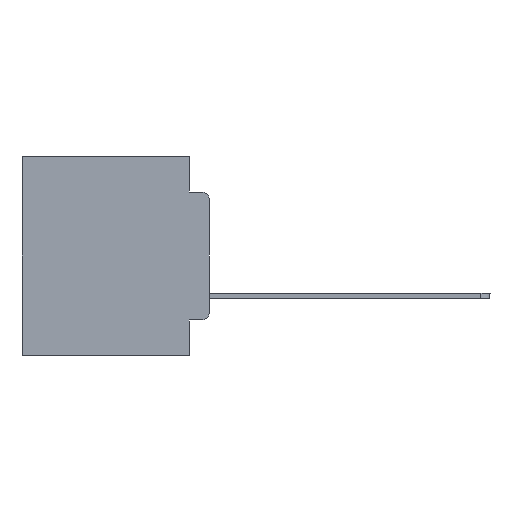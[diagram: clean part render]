
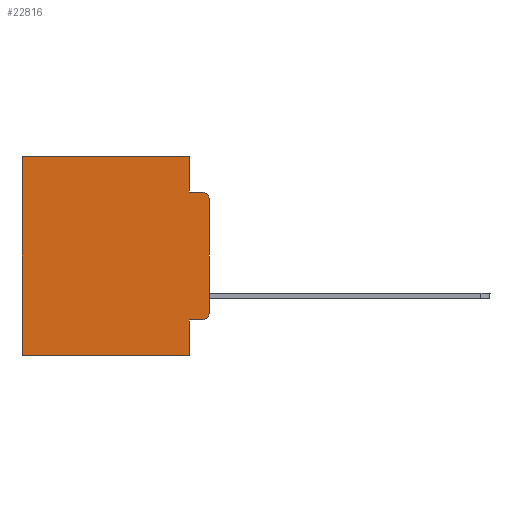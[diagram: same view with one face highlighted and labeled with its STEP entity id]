
A CAD part, left-side view. The second image highlights one B-rep face of the part: STEP entity #22816.
In plain terms, the highlighted planar face has unit normal (-1, 0, 0).
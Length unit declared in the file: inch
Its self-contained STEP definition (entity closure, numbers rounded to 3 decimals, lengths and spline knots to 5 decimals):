
#14 = CARTESIAN_POINT ( 'NONE',  ( 0.298, 0.051, 0. ) ) ;
#615 = VECTOR ( 'NONE', #640, 39.37008 ) ;
#640 = DIRECTION ( 'NONE',  ( 0., 0., -1. ) ) ;
#774 = CARTESIAN_POINT ( 'NONE',  ( 0.298, 0.051, -0.4115 ) ) ;
#1004 = LINE ( 'NONE', #8736, #21366 ) ;
#1030 = AXIS2_PLACEMENT_3D ( 'NONE', #10919, #24920, #16826 ) ;
#1544 = CARTESIAN_POINT ( 'NONE',  ( 0.298, 0., 0. ) ) ;
#1681 = DIRECTION ( 'NONE',  ( 0., 1., 0. ) ) ;
#2291 = CIRCLE ( 'NONE', #1030, 0.02 ) ;
#2389 = VECTOR ( 'NONE', #4589, 39.37008 ) ;
#2573 = LINE ( 'NONE', #18307, #615 ) ;
#3080 = VERTEX_POINT ( 'NONE', #11454 ) ;
#3164 = EDGE_CURVE ( 'NONE', #3080, #12887, #21614, .T. ) ;
#3200 = ORIENTED_EDGE ( 'NONE', *, *, #3164, .F. ) ;
#3314 = DIRECTION ( 'NONE',  ( 0., 0., -1. ) ) ;
#3626 = LINE ( 'NONE', #14, #10348 ) ;
#3738 = ORIENTED_EDGE ( 'NONE', *, *, #6364, .F. ) ;
#4007 = VECTOR ( 'NONE', #17377, 39.37008 ) ;
#4589 = DIRECTION ( 'NONE',  ( 0., 0., -1. ) ) ;
#6128 = VERTEX_POINT ( 'NONE', #24958 ) ;
#6364 = EDGE_CURVE ( 'NONE', #21092, #3080, #3626, .T. ) ;
#6742 = CARTESIAN_POINT ( 'NONE',  ( 0.298, 0., 0. ) ) ;
#7384 = EDGE_LOOP ( 'NONE', ( #25412, #16999, #7900, #16274, #13471, #11662, #3200, #3738, #22404, #22449 ) ) ;
#7455 = VERTEX_POINT ( 'NONE', #12932 ) ;
#7464 = VECTOR ( 'NONE', #1681, 39.37008 ) ;
#7879 = EDGE_CURVE ( 'NONE', #25225, #22087, #16377, .T. ) ;
#7900 = ORIENTED_EDGE ( 'NONE', *, *, #11359, .F. ) ;
#8012 = DIRECTION ( 'NONE',  ( 1., 0., 0. ) ) ;
#8187 = VERTEX_POINT ( 'NONE', #18287 ) ;
#8594 = DIRECTION ( 'NONE',  ( -1., 0., 0. ) ) ;
#8736 = CARTESIAN_POINT ( 'NONE',  ( 0.298, 0.051, -0.4115 ) ) ;
#9290 = EDGE_CURVE ( 'NONE', #25225, #8187, #10383, .T. ) ;
#9318 = VECTOR ( 'NONE', #20363, 39.37008 ) ;
#10348 = VECTOR ( 'NONE', #17791, 39.37008 ) ;
#10383 = LINE ( 'NONE', #18616, #2389 ) ;
#10919 = CARTESIAN_POINT ( 'NONE',  ( 0.298, 0.02, -0.3915 ) ) ;
#11359 = EDGE_CURVE ( 'NONE', #8187, #6128, #17929, .T. ) ;
#11454 = CARTESIAN_POINT ( 'NONE',  ( 0.298, 0.051, -0.5 ) ) ;
#11662 = ORIENTED_EDGE ( 'NONE', *, *, #20766, .T. ) ;
#11667 = EDGE_CURVE ( 'NONE', #7455, #18899, #21604, .T. ) ;
#12361 = VECTOR ( 'NONE', #22524, 39.37008 ) ;
#12363 = CARTESIAN_POINT ( 'NONE',  ( 0.298, 0.051, -0.0885 ) ) ;
#12887 = VERTEX_POINT ( 'NONE', #15535 ) ;
#12932 = CARTESIAN_POINT ( 'NONE',  ( 0.298, 0., -0.1085 ) ) ;
#13471 = ORIENTED_EDGE ( 'NONE', *, *, #7879, .T. ) ;
#13690 = CARTESIAN_POINT ( 'NONE',  ( 0.298, 0., -0.3915 ) ) ;
#13691 = FACE_OUTER_BOUND ( 'NONE', #7384, .T. ) ;
#14458 = EDGE_CURVE ( 'NONE', #21092, #17081, #1004, .T. ) ;
#15535 = CARTESIAN_POINT ( 'NONE',  ( 0.298, 0.473, -0.5 ) ) ;
#16274 = ORIENTED_EDGE ( 'NONE', *, *, #9290, .F. ) ;
#16324 = DIRECTION ( 'NONE',  ( 0., -1., 0. ) ) ;
#16377 = LINE ( 'NONE', #6742, #12361 ) ;
#16575 = CARTESIAN_POINT ( 'NONE',  ( 0.298, 0.02, -0.1085 ) ) ;
#16787 = CARTESIAN_POINT ( 'NONE',  ( 0.298, 0.473, 0. ) ) ;
#16826 = DIRECTION ( 'NONE',  ( 0., 0., -1. ) ) ;
#16999 = ORIENTED_EDGE ( 'NONE', *, *, #21706, .T. ) ;
#17081 = VERTEX_POINT ( 'NONE', #19128 ) ;
#17377 = DIRECTION ( 'NONE',  ( 0., 0., -1. ) ) ;
#17791 = DIRECTION ( 'NONE',  ( 0., 0., -1. ) ) ;
#17929 = LINE ( 'NONE', #12363, #9318 ) ;
#18287 = CARTESIAN_POINT ( 'NONE',  ( 0.298, 0.051, -0.0885 ) ) ;
#18307 = CARTESIAN_POINT ( 'NONE',  ( 0.298, 0.473, 0. ) ) ;
#18616 = CARTESIAN_POINT ( 'NONE',  ( 0.298, 0.051, 0. ) ) ;
#18899 = VERTEX_POINT ( 'NONE', #13690 ) ;
#19128 = CARTESIAN_POINT ( 'NONE',  ( 0.298, 0.02, -0.4115 ) ) ;
#19600 = PLANE ( 'NONE',  #23440 ) ;
#19726 = CARTESIAN_POINT ( 'NONE',  ( 0.298, 0., 0. ) ) ;
#19742 = CIRCLE ( 'NONE', #20146, 0.02 ) ;
#20146 = AXIS2_PLACEMENT_3D ( 'NONE', #16575, #8594, #3314 ) ;
#20363 = DIRECTION ( 'NONE',  ( 0., -1., 0. ) ) ;
#20766 = EDGE_CURVE ( 'NONE', #22087, #12887, #2573, .T. ) ;
#20873 = EDGE_CURVE ( 'NONE', #17081, #18899, #2291, .T. ) ;
#21092 = VERTEX_POINT ( 'NONE', #774 ) ;
#21355 = CARTESIAN_POINT ( 'NONE',  ( 0.298, 0., -0.5 ) ) ;
#21366 = VECTOR ( 'NONE', #16324, 39.37008 ) ;
#21524 = DIRECTION ( 'NONE',  ( 0., 0., -1. ) ) ;
#21604 = LINE ( 'NONE', #1544, #4007 ) ;
#21614 = LINE ( 'NONE', #21355, #7464 ) ;
#21706 = EDGE_CURVE ( 'NONE', #7455, #6128, #19742, .T. ) ;
#22087 = VERTEX_POINT ( 'NONE', #16787 ) ;
#22404 = ORIENTED_EDGE ( 'NONE', *, *, #14458, .T. ) ;
#22449 = ORIENTED_EDGE ( 'NONE', *, *, #20873, .T. ) ;
#22524 = DIRECTION ( 'NONE',  ( 0., 1., 0. ) ) ;
#22816 = ADVANCED_FACE ( 'NONE', ( #13691 ), #19600, .F. ) ;
#23330 = CARTESIAN_POINT ( 'NONE',  ( 0.298, 0.051, 0. ) ) ;
#23440 = AXIS2_PLACEMENT_3D ( 'NONE', #19726, #8012, #21524 ) ;
#24920 = DIRECTION ( 'NONE',  ( -1., 0., 0. ) ) ;
#24958 = CARTESIAN_POINT ( 'NONE',  ( 0.298, 0.02, -0.0885 ) ) ;
#25225 = VERTEX_POINT ( 'NONE', #23330 ) ;
#25412 = ORIENTED_EDGE ( 'NONE', *, *, #11667, .F. ) ;
